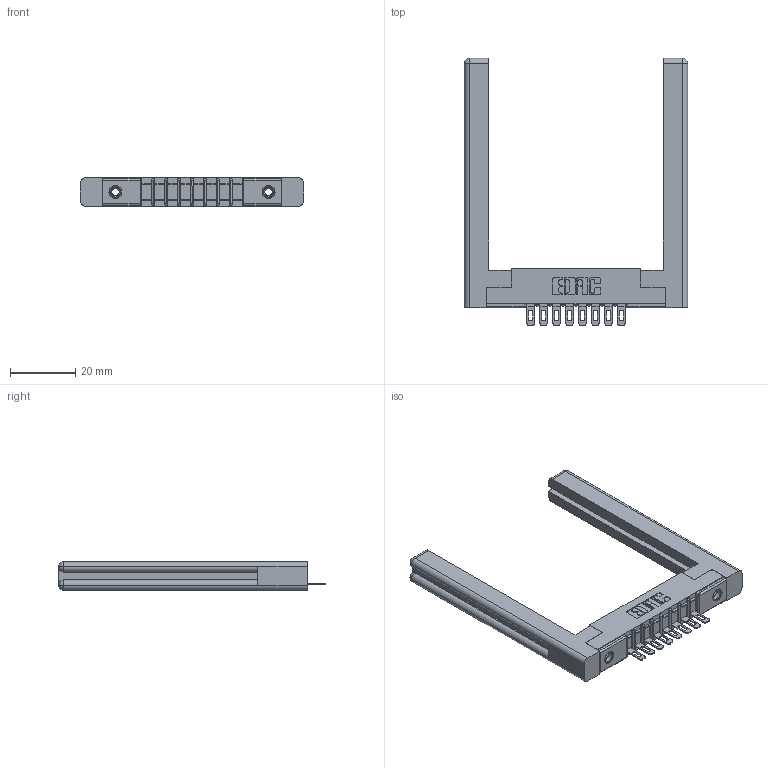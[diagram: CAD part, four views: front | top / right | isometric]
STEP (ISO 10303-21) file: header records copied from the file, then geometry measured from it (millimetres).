
FILE_DESCRIPTION (( 'STEP AP203' ), '1' );
FILE_NAME ('357-008-501-158.STEP', '2019-09-16T17:36:55', ( '' ), ( '' ), 'SwSTEP 2.0', 'SolidWorks 2016', '' );
FILE_SCHEMA (( 'CONFIG_CONTROL_DESIGN' ));
Length unit declared in the file: inch
Products named in the file (5): 307-220-058; 345-250-001_345-250-001-102; 307 Part_.156 Dia Mounting Holes; 357-008-501-158; 307-290-002_501
Assembly tree (13 placements, depth 2):
  357-008-501-158
    307 Part_.156 Dia Mounting Holes
    307-290-002_501  x8
    307-220-058  x2
    345-250-001_345-250-001-102  x2
Bounding box: 68.33 x 81.74 x 8.71 mm (x, y, z)
Volume: 12188.7 mm3; surface area: 12503.4 mm2
Topology: 13 solids, 13 shells, 877 faces, 2581 edges, 1682 vertices
Faces by surface type: plane 506, cylinder 329, sphere 18, torus 12, cone 12
Entity records: 14477 total; most frequent: CARTESIAN_POINT 2443, ORIENTED_EDGE 2372, DIRECTION 2354, EDGE_CURVE 1186, LINE 884, VECTOR 884, VERTEX_POINT 770, AXIS2_PLACEMENT_3D 735
